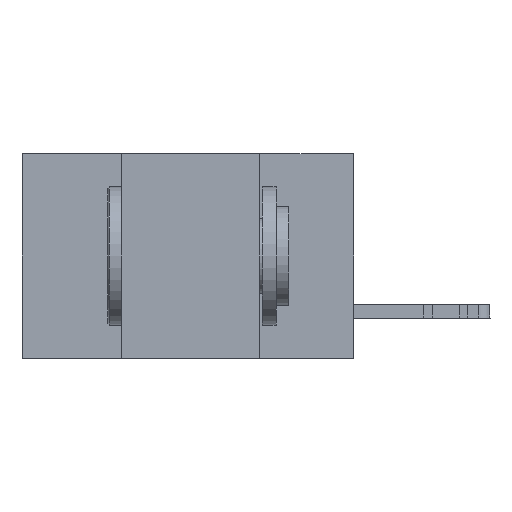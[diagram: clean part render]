
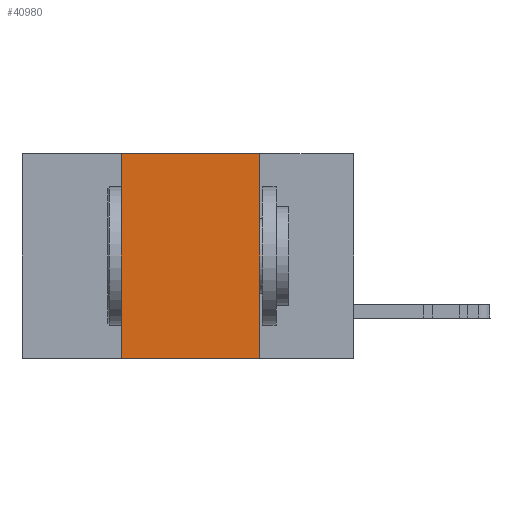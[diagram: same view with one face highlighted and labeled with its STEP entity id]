
A CAD part, left-side view. The second image highlights one B-rep face of the part: STEP entity #40980.
In plain terms, the highlighted planar face has unit normal (-1, 0, 0).
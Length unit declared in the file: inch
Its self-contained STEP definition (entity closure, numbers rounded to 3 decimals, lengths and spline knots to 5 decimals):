
#1513 = DIRECTION ( 'NONE',  ( 0., -1., 0. ) ) ;
#4536 = DIRECTION ( 'NONE',  ( 0., 0., -1. ) ) ;
#6208 = FACE_OUTER_BOUND ( 'NONE', #9632, .T. ) ;
#6584 = CARTESIAN_POINT ( 'NONE',  ( 0., 0.6, 0. ) ) ;
#8053 = VECTOR ( 'NONE', #1513, 39.37008 ) ;
#8270 = LINE ( 'NONE', #41851, #17810 ) ;
#9632 = EDGE_LOOP ( 'NONE', ( #17192, #41578, #16636, #20442 ) ) ;
#10250 = VERTEX_POINT ( 'NONE', #43281 ) ;
#13599 = DIRECTION ( 'NONE',  ( 0., 0., -1. ) ) ;
#16019 = DIRECTION ( 'NONE',  ( 0., 0., 1. ) ) ;
#16602 = DIRECTION ( 'NONE',  ( 1., 0., 0. ) ) ;
#16636 = ORIENTED_EDGE ( 'NONE', *, *, #40857, .F. ) ;
#17192 = ORIENTED_EDGE ( 'NONE', *, *, #33338, .F. ) ;
#17198 = VERTEX_POINT ( 'NONE', #33932 ) ;
#17810 = VECTOR ( 'NONE', #4536, 39.37008 ) ;
#19534 = EDGE_CURVE ( 'NONE', #26826, #40921, #26242, .T. ) ;
#20442 = ORIENTED_EDGE ( 'NONE', *, *, #19534, .T. ) ;
#20551 = VECTOR ( 'NONE', #16019, 39.37008 ) ;
#22100 = CARTESIAN_POINT ( 'NONE',  ( 0., 0.6, -0.37 ) ) ;
#22905 = CARTESIAN_POINT ( 'NONE',  ( 0., 0.42, 0. ) ) ;
#24143 = VECTOR ( 'NONE', #33227, 39.37008 ) ;
#26242 = LINE ( 'NONE', #22100, #8053 ) ;
#26444 = AXIS2_PLACEMENT_3D ( 'NONE', #40480, #16602, #13599 ) ;
#26492 = LINE ( 'NONE', #22905, #20551 ) ;
#26826 = VERTEX_POINT ( 'NONE', #37624 ) ;
#33227 = DIRECTION ( 'NONE',  ( 0., -1., 0. ) ) ;
#33338 = EDGE_CURVE ( 'NONE', #10250, #40921, #8270, .T. ) ;
#33404 = CARTESIAN_POINT ( 'NONE',  ( 0., 0.17, -0.37 ) ) ;
#33932 = CARTESIAN_POINT ( 'NONE',  ( 0., 0.42, 0. ) ) ;
#34084 = PLANE ( 'NONE',  #26444 ) ;
#34376 = EDGE_CURVE ( 'NONE', #17198, #10250, #37397, .T. ) ;
#37397 = LINE ( 'NONE', #6584, #24143 ) ;
#37624 = CARTESIAN_POINT ( 'NONE',  ( 0., 0.42, -0.37 ) ) ;
#40480 = CARTESIAN_POINT ( 'NONE',  ( 0., 0.6, 0. ) ) ;
#40857 = EDGE_CURVE ( 'NONE', #26826, #17198, #26492, .T. ) ;
#40921 = VERTEX_POINT ( 'NONE', #33404 ) ;
#40980 = ADVANCED_FACE ( 'NONE', ( #6208 ), #34084, .F. ) ;
#41578 = ORIENTED_EDGE ( 'NONE', *, *, #34376, .F. ) ;
#41851 = CARTESIAN_POINT ( 'NONE',  ( 0., 0.17, 0. ) ) ;
#43281 = CARTESIAN_POINT ( 'NONE',  ( 0., 0.17, 0. ) ) ;
